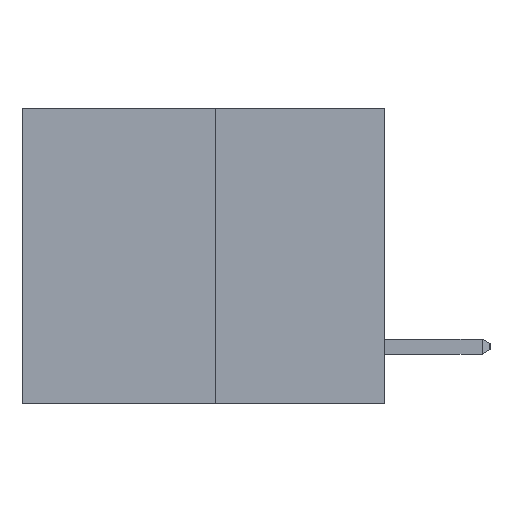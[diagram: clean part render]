
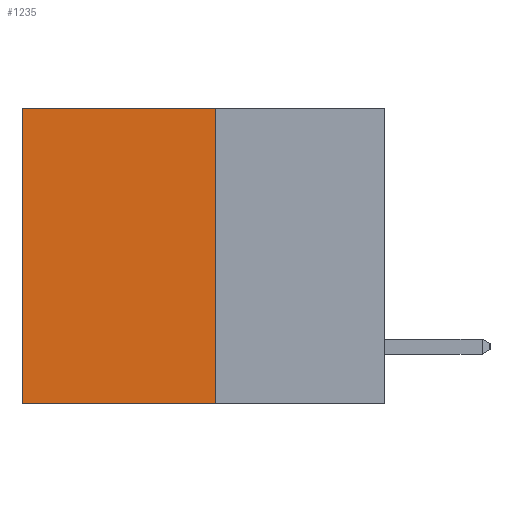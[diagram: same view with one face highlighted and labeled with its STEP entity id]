
A CAD part, left-side view. The second image highlights one B-rep face of the part: STEP entity #1235.
In plain terms, the highlighted planar face has unit normal (-1, 0, 0).
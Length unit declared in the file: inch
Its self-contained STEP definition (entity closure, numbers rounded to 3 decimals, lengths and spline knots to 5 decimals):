
#15 = VERTEX_POINT ( 'NONE', #12810 ) ;
#623 = DIRECTION ( 'NONE',  ( 0., 1., 0. ) ) ;
#640 = VERTEX_POINT ( 'NONE', #3965 ) ;
#788 = CARTESIAN_POINT ( 'NONE',  ( 0.3165, 0.6, -0.49 ) ) ;
#1235 = ADVANCED_FACE ( 'NONE', ( #8822 ), #6370, .F. ) ;
#1428 = LINE ( 'NONE', #8349, #2858 ) ;
#1691 = EDGE_CURVE ( 'NONE', #15, #640, #5625, .T. ) ;
#1887 = ORIENTED_EDGE ( 'NONE', *, *, #1691, .F. ) ;
#2858 = VECTOR ( 'NONE', #5330, 39.37008 ) ;
#2877 = LINE ( 'NONE', #788, #6684 ) ;
#3505 = EDGE_LOOP ( 'NONE', ( #4361, #7723, #1887, #7543 ) ) ;
#3818 = EDGE_CURVE ( 'NONE', #15, #12627, #1428, .T. ) ;
#3965 = CARTESIAN_POINT ( 'NONE',  ( 0.3165, 0.28, -0.49 ) ) ;
#4361 = ORIENTED_EDGE ( 'NONE', *, *, #12014, .T. ) ;
#4773 = VERTEX_POINT ( 'NONE', #7057 ) ;
#4927 = VECTOR ( 'NONE', #623, 39.37008 ) ;
#5330 = DIRECTION ( 'NONE',  ( 0., 1., 0. ) ) ;
#5625 = LINE ( 'NONE', #11272, #11190 ) ;
#6310 = LINE ( 'NONE', #6691, #4927 ) ;
#6370 = PLANE ( 'NONE',  #9331 ) ;
#6684 = VECTOR ( 'NONE', #7128, 39.37008 ) ;
#6691 = CARTESIAN_POINT ( 'NONE',  ( 0.3165, 0.28, -0.49 ) ) ;
#7057 = CARTESIAN_POINT ( 'NONE',  ( 0.3165, 0.6, -0.49 ) ) ;
#7128 = DIRECTION ( 'NONE',  ( 0., 0., -1. ) ) ;
#7275 = CARTESIAN_POINT ( 'NONE',  ( 0.3165, 0.28, -0.49 ) ) ;
#7408 = DIRECTION ( 'NONE',  ( 0., 0., -1. ) ) ;
#7543 = ORIENTED_EDGE ( 'NONE', *, *, #3818, .T. ) ;
#7723 = ORIENTED_EDGE ( 'NONE', *, *, #9900, .F. ) ;
#8271 = DIRECTION ( 'NONE',  ( 0., 0., -1. ) ) ;
#8349 = CARTESIAN_POINT ( 'NONE',  ( 0.3165, 0.28, 0. ) ) ;
#8412 = DIRECTION ( 'NONE',  ( 1., 0., 0. ) ) ;
#8822 = FACE_OUTER_BOUND ( 'NONE', #3505, .T. ) ;
#9331 = AXIS2_PLACEMENT_3D ( 'NONE', #7275, #8412, #7408 ) ;
#9900 = EDGE_CURVE ( 'NONE', #640, #4773, #6310, .T. ) ;
#10808 = CARTESIAN_POINT ( 'NONE',  ( 0.3165, 0.6, 0. ) ) ;
#11190 = VECTOR ( 'NONE', #8271, 39.37008 ) ;
#11272 = CARTESIAN_POINT ( 'NONE',  ( 0.3165, 0.28, -0.49 ) ) ;
#12014 = EDGE_CURVE ( 'NONE', #12627, #4773, #2877, .T. ) ;
#12627 = VERTEX_POINT ( 'NONE', #10808 ) ;
#12810 = CARTESIAN_POINT ( 'NONE',  ( 0.3165, 0.28, 0. ) ) ;
